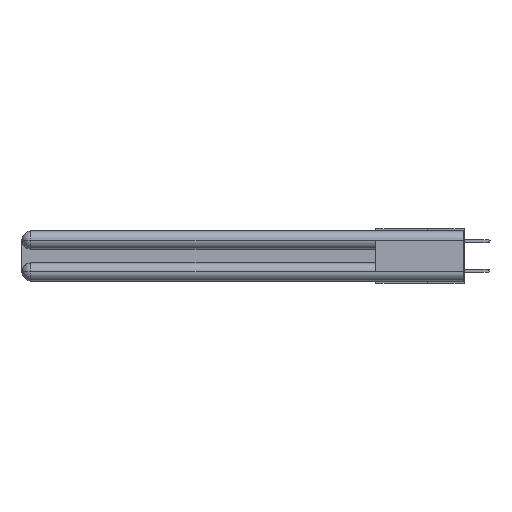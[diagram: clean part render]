
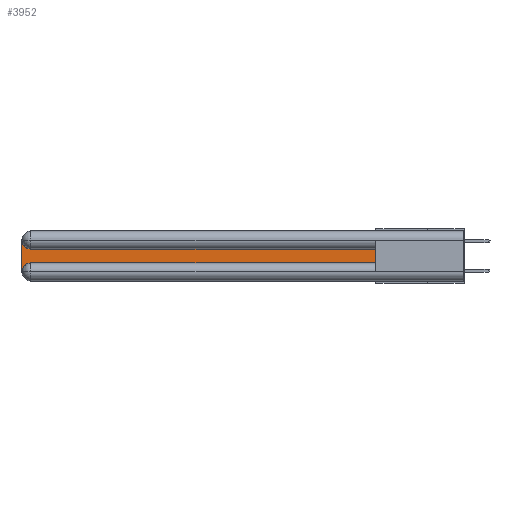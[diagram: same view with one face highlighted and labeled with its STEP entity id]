
A CAD part, left-side view. The second image highlights one B-rep face of the part: STEP entity #3952.
In plain terms, the highlighted planar face has unit normal (-1, 0, 0).
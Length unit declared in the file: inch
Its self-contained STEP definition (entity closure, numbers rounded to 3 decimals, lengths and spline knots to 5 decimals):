
#566 = CARTESIAN_POINT ( 'NONE',  ( 0.075, 0.6, -0.2175 ) ) ;
#867 = CARTESIAN_POINT ( 'NONE',  ( 0.075, 3., -0.2775 ) ) ;
#971 = CARTESIAN_POINT ( 'NONE',  ( 0.075, 2.94, -0.1225 ) ) ;
#985 = AXIS2_PLACEMENT_3D ( 'NONE', #5582, #13652, #25516 ) ;
#1503 = LINE ( 'NONE', #25262, #13688 ) ;
#1587 = EDGE_CURVE ( 'NONE', #17626, #6065, #3484, .T. ) ;
#2627 = ORIENTED_EDGE ( 'NONE', *, *, #18311, .T. ) ;
#2796 = DIRECTION ( 'NONE',  ( 0., 0., -1. ) ) ;
#3484 = LINE ( 'NONE', #30284, #28531 ) ;
#3952 = ADVANCED_FACE ( 'NONE', ( #13070 ), #24665, .F. ) ;
#4492 = ORIENTED_EDGE ( 'NONE', *, *, #1587, .T. ) ;
#5582 = CARTESIAN_POINT ( 'NONE',  ( 0.075, 2.94, -0.0625 ) ) ;
#5930 = ORIENTED_EDGE ( 'NONE', *, *, #19551, .T. ) ;
#6065 = VERTEX_POINT ( 'NONE', #566 ) ;
#6764 = CIRCLE ( 'NONE', #8717, 0.06 ) ;
#7790 = LINE ( 'NONE', #14213, #29058 ) ;
#8063 = ORIENTED_EDGE ( 'NONE', *, *, #30876, .T. ) ;
#8717 = AXIS2_PLACEMENT_3D ( 'NONE', #14104, #18954, #26271 ) ;
#8792 = VERTEX_POINT ( 'NONE', #971 ) ;
#13070 = FACE_OUTER_BOUND ( 'NONE', #16437, .T. ) ;
#13652 = DIRECTION ( 'NONE',  ( 1., 0., 0. ) ) ;
#13688 = VECTOR ( 'NONE', #18395, 39.37008 ) ;
#14104 = CARTESIAN_POINT ( 'NONE',  ( 0.075, 2.94, -0.2775 ) ) ;
#14213 = CARTESIAN_POINT ( 'NONE',  ( 0.075, 3., -0.2175 ) ) ;
#15204 = AXIS2_PLACEMENT_3D ( 'NONE', #27207, #29525, #2796 ) ;
#15689 = CARTESIAN_POINT ( 'NONE',  ( 0.075, 0.6, -0.1225 ) ) ;
#16437 = EDGE_LOOP ( 'NONE', ( #29559, #26147, #5930, #2627, #4492, #8063 ) ) ;
#17626 = VERTEX_POINT ( 'NONE', #17680 ) ;
#17680 = CARTESIAN_POINT ( 'NONE',  ( 0.075, 2.94, -0.2175 ) ) ;
#18067 = CARTESIAN_POINT ( 'NONE',  ( 0.075, 0.6, -0.1225 ) ) ;
#18241 = DIRECTION ( 'NONE',  ( 0., -1., 0. ) ) ;
#18311 = EDGE_CURVE ( 'NONE', #20537, #17626, #6764, .T. ) ;
#18395 = DIRECTION ( 'NONE',  ( 0., 0., 1. ) ) ;
#18954 = DIRECTION ( 'NONE',  ( 1., 0., 0. ) ) ;
#19551 = EDGE_CURVE ( 'NONE', #28061, #20537, #7790, .T. ) ;
#20196 = DIRECTION ( 'NONE',  ( 0., 1., 0. ) ) ;
#20537 = VERTEX_POINT ( 'NONE', #867 ) ;
#20918 = CARTESIAN_POINT ( 'NONE',  ( 0.075, 3., -0.0625 ) ) ;
#21729 = EDGE_CURVE ( 'NONE', #8792, #28061, #23105, .T. ) ;
#21830 = VERTEX_POINT ( 'NONE', #15689 ) ;
#22089 = EDGE_CURVE ( 'NONE', #21830, #8792, #29108, .T. ) ;
#23105 = CIRCLE ( 'NONE', #985, 0.06 ) ;
#24665 = PLANE ( 'NONE',  #15204 ) ;
#25262 = CARTESIAN_POINT ( 'NONE',  ( 0.075, 0.6, -0.2175 ) ) ;
#25516 = DIRECTION ( 'NONE',  ( 0., 0., -1. ) ) ;
#26147 = ORIENTED_EDGE ( 'NONE', *, *, #21729, .T. ) ;
#26271 = DIRECTION ( 'NONE',  ( 0., 0., -1. ) ) ;
#27207 = CARTESIAN_POINT ( 'NONE',  ( 0.075, 3., -0.1225 ) ) ;
#28061 = VERTEX_POINT ( 'NONE', #20918 ) ;
#28531 = VECTOR ( 'NONE', #18241, 39.37008 ) ;
#28996 = DIRECTION ( 'NONE',  ( 0., 0., -1. ) ) ;
#29058 = VECTOR ( 'NONE', #28996, 39.37008 ) ;
#29108 = LINE ( 'NONE', #18067, #30630 ) ;
#29525 = DIRECTION ( 'NONE',  ( 1., 0., 0. ) ) ;
#29559 = ORIENTED_EDGE ( 'NONE', *, *, #22089, .T. ) ;
#30284 = CARTESIAN_POINT ( 'NONE',  ( 0.075, 0.6, -0.2175 ) ) ;
#30630 = VECTOR ( 'NONE', #20196, 39.37008 ) ;
#30876 = EDGE_CURVE ( 'NONE', #6065, #21830, #1503, .T. ) ;
